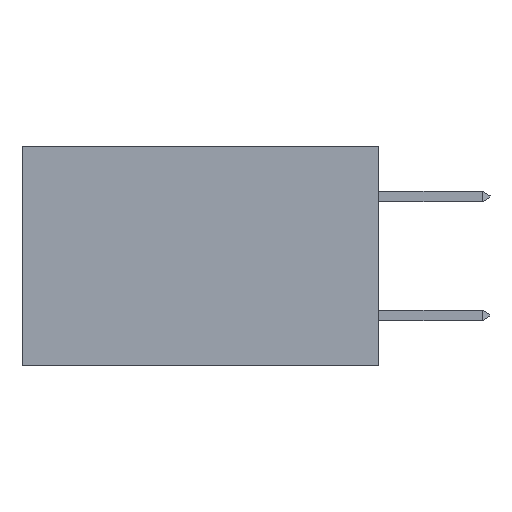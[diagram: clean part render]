
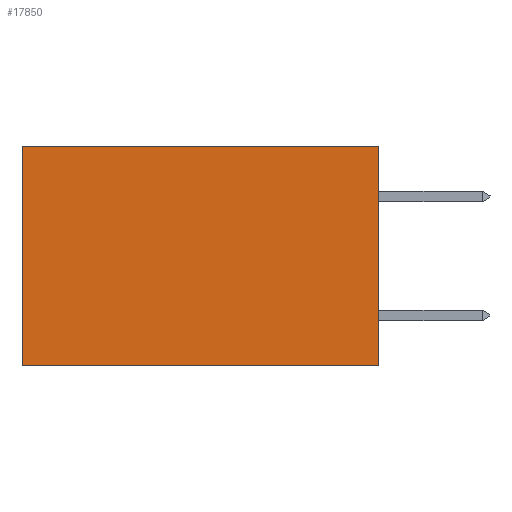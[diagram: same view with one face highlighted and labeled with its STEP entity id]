
A CAD part, left-side view. The second image highlights one B-rep face of the part: STEP entity #17850.
In plain terms, the highlighted planar face has unit normal (-1, 0, 0).
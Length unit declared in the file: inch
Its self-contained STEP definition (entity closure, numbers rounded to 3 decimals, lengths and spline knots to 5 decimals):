
#56 = LINE ( 'NONE', #16355, #16717 ) ;
#72 = CARTESIAN_POINT ( 'NONE',  ( 0.2615, 0., -0.37 ) ) ;
#871 = DIRECTION ( 'NONE',  ( 1., 0., 0. ) ) ;
#2042 = VECTOR ( 'NONE', #8142, 39.37008 ) ;
#2741 = EDGE_LOOP ( 'NONE', ( #16758, #15593, #19192, #18757 ) ) ;
#3689 = EDGE_CURVE ( 'NONE', #10610, #5856, #9363, .T. ) ;
#4305 = LINE ( 'NONE', #72, #2042 ) ;
#4765 = LINE ( 'NONE', #17842, #17379 ) ;
#5531 = PLANE ( 'NONE',  #20256 ) ;
#5666 = EDGE_CURVE ( 'NONE', #10610, #9694, #4765, .T. ) ;
#5856 = VERTEX_POINT ( 'NONE', #12235 ) ;
#6238 = DIRECTION ( 'NONE',  ( 0., 1., 0. ) ) ;
#6492 = EDGE_CURVE ( 'NONE', #5856, #8192, #56, .T. ) ;
#8142 = DIRECTION ( 'NONE',  ( 0., 1., 0. ) ) ;
#8192 = VERTEX_POINT ( 'NONE', #13745 ) ;
#8800 = DIRECTION ( 'NONE',  ( 0., 0., -1. ) ) ;
#9363 = LINE ( 'NONE', #15900, #11060 ) ;
#9694 = VERTEX_POINT ( 'NONE', #10559 ) ;
#9853 = DIRECTION ( 'NONE',  ( 0., 0., -1. ) ) ;
#10559 = CARTESIAN_POINT ( 'NONE',  ( 0.2615, 0., -0.37 ) ) ;
#10610 = VERTEX_POINT ( 'NONE', #13536 ) ;
#11060 = VECTOR ( 'NONE', #6238, 39.37008 ) ;
#12168 = CARTESIAN_POINT ( 'NONE',  ( 0.2615, 0., -0.37 ) ) ;
#12235 = CARTESIAN_POINT ( 'NONE',  ( 0.2615, 0.6, 0. ) ) ;
#12394 = FACE_OUTER_BOUND ( 'NONE', #2741, .T. ) ;
#13372 = EDGE_CURVE ( 'NONE', #9694, #8192, #4305, .T. ) ;
#13536 = CARTESIAN_POINT ( 'NONE',  ( 0.2615, 0., 0. ) ) ;
#13745 = CARTESIAN_POINT ( 'NONE',  ( 0.2615, 0.6, -0.37 ) ) ;
#15593 = ORIENTED_EDGE ( 'NONE', *, *, #13372, .F. ) ;
#15900 = CARTESIAN_POINT ( 'NONE',  ( 0.2615, 0., 0. ) ) ;
#16355 = CARTESIAN_POINT ( 'NONE',  ( 0.2615, 0.6, -0.37 ) ) ;
#16717 = VECTOR ( 'NONE', #9853, 39.37008 ) ;
#16758 = ORIENTED_EDGE ( 'NONE', *, *, #6492, .T. ) ;
#16903 = DIRECTION ( 'NONE',  ( 0., 0., -1. ) ) ;
#17379 = VECTOR ( 'NONE', #8800, 39.37008 ) ;
#17842 = CARTESIAN_POINT ( 'NONE',  ( 0.2615, 0., -0.37 ) ) ;
#17850 = ADVANCED_FACE ( 'NONE', ( #12394 ), #5531, .F. ) ;
#18757 = ORIENTED_EDGE ( 'NONE', *, *, #3689, .T. ) ;
#19192 = ORIENTED_EDGE ( 'NONE', *, *, #5666, .F. ) ;
#20256 = AXIS2_PLACEMENT_3D ( 'NONE', #12168, #871, #16903 ) ;
